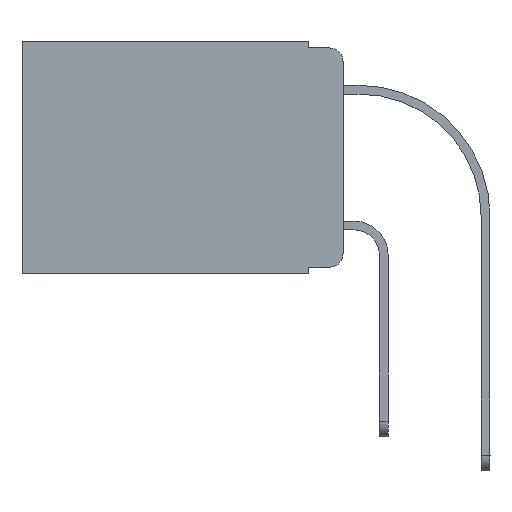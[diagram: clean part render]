
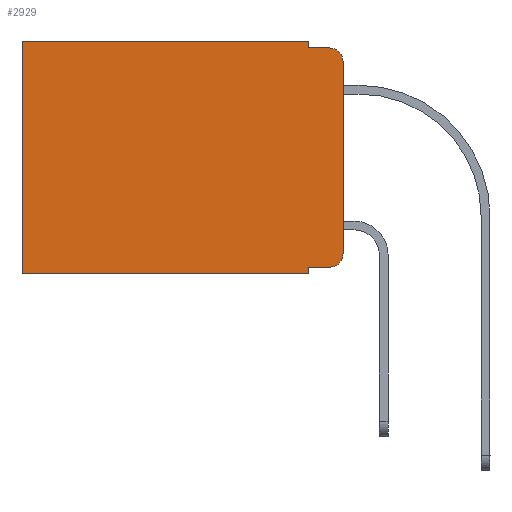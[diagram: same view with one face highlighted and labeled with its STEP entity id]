
A CAD part, left-side view. The second image highlights one B-rep face of the part: STEP entity #2929.
In plain terms, the highlighted planar face has unit normal (-1, 0, 0).
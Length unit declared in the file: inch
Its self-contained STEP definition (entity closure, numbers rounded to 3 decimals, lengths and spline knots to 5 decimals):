
#18 = DIRECTION ( 'NONE',  ( 0., 1., 0. ) ) ;
#55 = EDGE_CURVE ( 'NONE', #11567, #12426, #11790, .T. ) ;
#102 = DIRECTION ( 'NONE',  ( 0., 0., -1. ) ) ;
#237 = ORIENTED_EDGE ( 'NONE', *, *, #6909, .F. ) ;
#604 = LINE ( 'NONE', #14927, #2059 ) ;
#672 = VERTEX_POINT ( 'NONE', #4211 ) ;
#845 = CARTESIAN_POINT ( 'NONE',  ( 0.298, 0., -0.313 ) ) ;
#863 = CIRCLE ( 'NONE', #14184, 0.02 ) ;
#957 = CARTESIAN_POINT ( 'NONE',  ( 0.298, 0.02, -0.03 ) ) ;
#1061 = ORIENTED_EDGE ( 'NONE', *, *, #13654, .T. ) ;
#1064 = DIRECTION ( 'NONE',  ( 0., 0., -1. ) ) ;
#1068 = ORIENTED_EDGE ( 'NONE', *, *, #55, .F. ) ;
#1147 = LINE ( 'NONE', #10755, #7651 ) ;
#1747 = VERTEX_POINT ( 'NONE', #8754 ) ;
#2059 = VECTOR ( 'NONE', #14773, 39.37008 ) ;
#2246 = EDGE_CURVE ( 'NONE', #5381, #13109, #2525, .T. ) ;
#2421 = DIRECTION ( 'NONE',  ( 0., -1., 0. ) ) ;
#2468 = FACE_OUTER_BOUND ( 'NONE', #9044, .T. ) ;
#2474 = EDGE_CURVE ( 'NONE', #11567, #1747, #9377, .T. ) ;
#2525 = LINE ( 'NONE', #7487, #10455 ) ;
#2806 = VECTOR ( 'NONE', #5823, 39.37008 ) ;
#2929 = ADVANCED_FACE ( 'NONE', ( #2468 ), #8296, .F. ) ;
#3070 = CARTESIAN_POINT ( 'NONE',  ( 0.298, 0.051, -0.333 ) ) ;
#3433 = LINE ( 'NONE', #7039, #6037 ) ;
#3732 = LINE ( 'NONE', #8372, #8415 ) ;
#3860 = ORIENTED_EDGE ( 'NONE', *, *, #2246, .F. ) ;
#4211 = CARTESIAN_POINT ( 'NONE',  ( 0.298, 0.051, -0.01 ) ) ;
#4977 = ORIENTED_EDGE ( 'NONE', *, *, #9035, .T. ) ;
#5381 = VERTEX_POINT ( 'NONE', #3070 ) ;
#5646 = LINE ( 'NONE', #10446, #9338 ) ;
#5648 = CARTESIAN_POINT ( 'NONE',  ( 0.298, 0.473, -0.343 ) ) ;
#5823 = DIRECTION ( 'NONE',  ( 0., 0., -1. ) ) ;
#5885 = CARTESIAN_POINT ( 'NONE',  ( 0.298, 0.02, -0.313 ) ) ;
#6037 = VECTOR ( 'NONE', #1064, 39.37008 ) ;
#6237 = DIRECTION ( 'NONE',  ( 0., 0., -1. ) ) ;
#6371 = ORIENTED_EDGE ( 'NONE', *, *, #15266, .F. ) ;
#6676 = ORIENTED_EDGE ( 'NONE', *, *, #8106, .T. ) ;
#6909 = EDGE_CURVE ( 'NONE', #12902, #672, #3433, .T. ) ;
#7033 = CARTESIAN_POINT ( 'NONE',  ( 0.298, 0.051, 0. ) ) ;
#7039 = CARTESIAN_POINT ( 'NONE',  ( 0.298, 0.051, 0. ) ) ;
#7263 = CARTESIAN_POINT ( 'NONE',  ( 0.298, 0., 0. ) ) ;
#7487 = CARTESIAN_POINT ( 'NONE',  ( 0.298, 0.051, 0. ) ) ;
#7651 = VECTOR ( 'NONE', #12013, 39.37008 ) ;
#8106 = EDGE_CURVE ( 'NONE', #12902, #13845, #5646, .T. ) ;
#8296 = PLANE ( 'NONE',  #15430 ) ;
#8372 = CARTESIAN_POINT ( 'NONE',  ( 0.298, 0., -0.343 ) ) ;
#8415 = VECTOR ( 'NONE', #18, 39.37008 ) ;
#8526 = DIRECTION ( 'NONE',  ( 1., 0., 0. ) ) ;
#8754 = CARTESIAN_POINT ( 'NONE',  ( 0.298, 0.02, -0.01 ) ) ;
#9035 = EDGE_CURVE ( 'NONE', #5381, #15330, #14615, .T. ) ;
#9044 = EDGE_LOOP ( 'NONE', ( #1068, #12749, #6371, #237, #6676, #15444, #9111, #3860, #4977, #1061 ) ) ;
#9111 = ORIENTED_EDGE ( 'NONE', *, *, #12909, .F. ) ;
#9258 = DIRECTION ( 'NONE',  ( 0., 1., 0. ) ) ;
#9338 = VECTOR ( 'NONE', #9258, 39.37008 ) ;
#9362 = VERTEX_POINT ( 'NONE', #5648 ) ;
#9377 = CIRCLE ( 'NONE', #10886, 0.02 ) ;
#9415 = DIRECTION ( 'NONE',  ( -1., 0., 0. ) ) ;
#9504 = CARTESIAN_POINT ( 'NONE',  ( 0.298, 0., 0. ) ) ;
#9647 = CARTESIAN_POINT ( 'NONE',  ( 0.298, 0.473, 0. ) ) ;
#9941 = CARTESIAN_POINT ( 'NONE',  ( 0.298, 0.051, -0.343 ) ) ;
#10446 = CARTESIAN_POINT ( 'NONE',  ( 0.298, 0., 0. ) ) ;
#10455 = VECTOR ( 'NONE', #6237, 39.37008 ) ;
#10737 = CARTESIAN_POINT ( 'NONE',  ( 0.298, 0., -0.03 ) ) ;
#10755 = CARTESIAN_POINT ( 'NONE',  ( 0.298, 0.473, 0. ) ) ;
#10886 = AXIS2_PLACEMENT_3D ( 'NONE', #957, #15426, #11890 ) ;
#11567 = VERTEX_POINT ( 'NONE', #10737 ) ;
#11790 = LINE ( 'NONE', #9504, #2806 ) ;
#11890 = DIRECTION ( 'NONE',  ( 0., 0., -1. ) ) ;
#12013 = DIRECTION ( 'NONE',  ( 0., 0., -1. ) ) ;
#12426 = VERTEX_POINT ( 'NONE', #845 ) ;
#12576 = EDGE_CURVE ( 'NONE', #13845, #9362, #1147, .T. ) ;
#12749 = ORIENTED_EDGE ( 'NONE', *, *, #2474, .T. ) ;
#12902 = VERTEX_POINT ( 'NONE', #7033 ) ;
#12909 = EDGE_CURVE ( 'NONE', #13109, #9362, #3732, .T. ) ;
#13109 = VERTEX_POINT ( 'NONE', #9941 ) ;
#13522 = CARTESIAN_POINT ( 'NONE',  ( 0.298, 0.051, -0.333 ) ) ;
#13603 = CARTESIAN_POINT ( 'NONE',  ( 0.298, 0.02, -0.333 ) ) ;
#13654 = EDGE_CURVE ( 'NONE', #15330, #12426, #863, .T. ) ;
#13845 = VERTEX_POINT ( 'NONE', #9647 ) ;
#14102 = VECTOR ( 'NONE', #2421, 39.37008 ) ;
#14184 = AXIS2_PLACEMENT_3D ( 'NONE', #5885, #9415, #15399 ) ;
#14615 = LINE ( 'NONE', #13522, #14102 ) ;
#14773 = DIRECTION ( 'NONE',  ( 0., -1., 0. ) ) ;
#14927 = CARTESIAN_POINT ( 'NONE',  ( 0.298, 0.051, -0.01 ) ) ;
#15266 = EDGE_CURVE ( 'NONE', #672, #1747, #604, .T. ) ;
#15330 = VERTEX_POINT ( 'NONE', #13603 ) ;
#15399 = DIRECTION ( 'NONE',  ( 0., 0., -1. ) ) ;
#15426 = DIRECTION ( 'NONE',  ( -1., 0., 0. ) ) ;
#15430 = AXIS2_PLACEMENT_3D ( 'NONE', #7263, #8526, #102 ) ;
#15444 = ORIENTED_EDGE ( 'NONE', *, *, #12576, .T. ) ;
